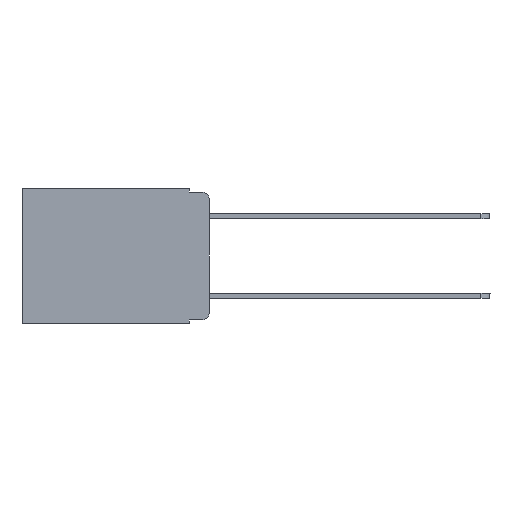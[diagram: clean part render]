
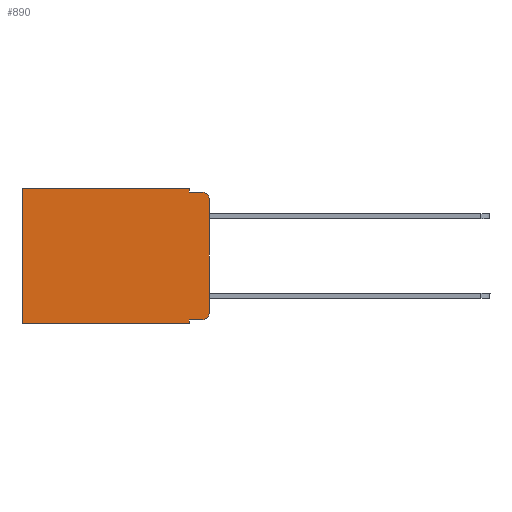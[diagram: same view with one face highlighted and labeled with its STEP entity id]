
A CAD part, left-side view. The second image highlights one B-rep face of the part: STEP entity #890.
In plain terms, the highlighted planar face has unit normal (-1, 0, 0).
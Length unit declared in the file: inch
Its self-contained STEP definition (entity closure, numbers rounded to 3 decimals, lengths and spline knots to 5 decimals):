
#130 = VERTEX_POINT ( 'NONE', #11338 ) ;
#194 = EDGE_CURVE ( 'NONE', #1970, #130, #1797, .T. ) ;
#262 = CARTESIAN_POINT ( 'NONE',  ( 0.298, 0.051, -0.01 ) ) ;
#366 = CARTESIAN_POINT ( 'NONE',  ( 0.298, 0.02, -0.333 ) ) ;
#757 = CARTESIAN_POINT ( 'NONE',  ( 0.298, 0.02, -0.03 ) ) ;
#767 = AXIS2_PLACEMENT_3D ( 'NONE', #757, #12430, #4545 ) ;
#769 = VERTEX_POINT ( 'NONE', #12163 ) ;
#771 = EDGE_CURVE ( 'NONE', #1970, #4406, #1932, .T. ) ;
#853 = CARTESIAN_POINT ( 'NONE',  ( 0.298, 0.051, -0.333 ) ) ;
#890 = ADVANCED_FACE ( 'NONE', ( #1318 ), #4174, .F. ) ;
#947 = ORIENTED_EDGE ( 'NONE', *, *, #4302, .F. ) ;
#1174 = VERTEX_POINT ( 'NONE', #366 ) ;
#1262 = EDGE_CURVE ( 'NONE', #769, #4809, #11128, .T. ) ;
#1296 = DIRECTION ( 'NONE',  ( 1., 0., 0. ) ) ;
#1318 = FACE_OUTER_BOUND ( 'NONE', #2190, .T. ) ;
#1337 = DIRECTION ( 'NONE',  ( 0., -1., 0. ) ) ;
#1653 = DIRECTION ( 'NONE',  ( 0., 0., -1. ) ) ;
#1671 = CARTESIAN_POINT ( 'NONE',  ( 0.298, 0.051, -0.333 ) ) ;
#1688 = CARTESIAN_POINT ( 'NONE',  ( 0.298, 0.051, 0. ) ) ;
#1797 = CIRCLE ( 'NONE', #767, 0.02 ) ;
#1932 = LINE ( 'NONE', #9241, #8735 ) ;
#1970 = VERTEX_POINT ( 'NONE', #4119 ) ;
#1990 = ORIENTED_EDGE ( 'NONE', *, *, #4877, .T. ) ;
#2064 = DIRECTION ( 'NONE',  ( 0., 0., -1. ) ) ;
#2074 = EDGE_CURVE ( 'NONE', #4519, #8644, #9302, .T. ) ;
#2190 = EDGE_LOOP ( 'NONE', ( #9070, #6346, #947, #5321, #1990, #2446, #9105, #8401, #3474, #5586 ) ) ;
#2446 = ORIENTED_EDGE ( 'NONE', *, *, #2074, .T. ) ;
#2481 = CARTESIAN_POINT ( 'NONE',  ( 0.298, 0.051, -0.01 ) ) ;
#2931 = CARTESIAN_POINT ( 'NONE',  ( 0.298, 0., 0. ) ) ;
#3101 = VECTOR ( 'NONE', #9969, 39.37008 ) ;
#3474 = ORIENTED_EDGE ( 'NONE', *, *, #5891, .T. ) ;
#4039 = DIRECTION ( 'NONE',  ( 0., 1., 0. ) ) ;
#4119 = CARTESIAN_POINT ( 'NONE',  ( 0.298, 0., -0.03 ) ) ;
#4174 = PLANE ( 'NONE',  #6075 ) ;
#4302 = EDGE_CURVE ( 'NONE', #4809, #130, #10733, .T. ) ;
#4406 = VERTEX_POINT ( 'NONE', #6830 ) ;
#4420 = DIRECTION ( 'NONE',  ( 0., 0., -1. ) ) ;
#4519 = VERTEX_POINT ( 'NONE', #7406 ) ;
#4545 = DIRECTION ( 'NONE',  ( 0., 0., -1. ) ) ;
#4728 = CARTESIAN_POINT ( 'NONE',  ( 0.298, 0.02, -0.313 ) ) ;
#4809 = VERTEX_POINT ( 'NONE', #262 ) ;
#4877 = EDGE_CURVE ( 'NONE', #769, #4519, #11783, .T. ) ;
#5139 = VERTEX_POINT ( 'NONE', #853 ) ;
#5321 = ORIENTED_EDGE ( 'NONE', *, *, #1262, .F. ) ;
#5505 = DIRECTION ( 'NONE',  ( 0., -1., 0. ) ) ;
#5561 = LINE ( 'NONE', #1688, #10544 ) ;
#5586 = ORIENTED_EDGE ( 'NONE', *, *, #9792, .T. ) ;
#5710 = CIRCLE ( 'NONE', #6623, 0.02 ) ;
#5865 = VECTOR ( 'NONE', #5505, 39.37008 ) ;
#5891 = EDGE_CURVE ( 'NONE', #5139, #1174, #10093, .T. ) ;
#5900 = CARTESIAN_POINT ( 'NONE',  ( 0.298, 0.051, 0. ) ) ;
#6075 = AXIS2_PLACEMENT_3D ( 'NONE', #2931, #1296, #2064 ) ;
#6346 = ORIENTED_EDGE ( 'NONE', *, *, #194, .T. ) ;
#6623 = AXIS2_PLACEMENT_3D ( 'NONE', #4728, #12495, #11435 ) ;
#6828 = VECTOR ( 'NONE', #1337, 39.37008 ) ;
#6830 = CARTESIAN_POINT ( 'NONE',  ( 0.298, 0., -0.313 ) ) ;
#7376 = VECTOR ( 'NONE', #8666, 39.37008 ) ;
#7406 = CARTESIAN_POINT ( 'NONE',  ( 0.298, 0.473, 0. ) ) ;
#8332 = DIRECTION ( 'NONE',  ( 0., 0., -1. ) ) ;
#8345 = CARTESIAN_POINT ( 'NONE',  ( 0.298, 0.051, -0.343 ) ) ;
#8401 = ORIENTED_EDGE ( 'NONE', *, *, #9256, .F. ) ;
#8502 = CARTESIAN_POINT ( 'NONE',  ( 0.298, 0.473, -0.343 ) ) ;
#8589 = VERTEX_POINT ( 'NONE', #8345 ) ;
#8644 = VERTEX_POINT ( 'NONE', #8502 ) ;
#8666 = DIRECTION ( 'NONE',  ( 0., 0., -1. ) ) ;
#8735 = VECTOR ( 'NONE', #1653, 39.37008 ) ;
#8901 = CARTESIAN_POINT ( 'NONE',  ( 0.298, 0., 0. ) ) ;
#9070 = ORIENTED_EDGE ( 'NONE', *, *, #771, .F. ) ;
#9105 = ORIENTED_EDGE ( 'NONE', *, *, #10756, .F. ) ;
#9241 = CARTESIAN_POINT ( 'NONE',  ( 0.298, 0., 0. ) ) ;
#9256 = EDGE_CURVE ( 'NONE', #5139, #8589, #5561, .T. ) ;
#9302 = LINE ( 'NONE', #9944, #11575 ) ;
#9450 = LINE ( 'NONE', #10900, #3101 ) ;
#9792 = EDGE_CURVE ( 'NONE', #1174, #4406, #5710, .T. ) ;
#9944 = CARTESIAN_POINT ( 'NONE',  ( 0.298, 0.473, 0. ) ) ;
#9969 = DIRECTION ( 'NONE',  ( 0., 1., 0. ) ) ;
#10093 = LINE ( 'NONE', #1671, #5865 ) ;
#10269 = VECTOR ( 'NONE', #4039, 39.37008 ) ;
#10544 = VECTOR ( 'NONE', #8332, 39.37008 ) ;
#10733 = LINE ( 'NONE', #2481, #6828 ) ;
#10756 = EDGE_CURVE ( 'NONE', #8589, #8644, #9450, .T. ) ;
#10900 = CARTESIAN_POINT ( 'NONE',  ( 0.298, 0., -0.343 ) ) ;
#11128 = LINE ( 'NONE', #5900, #7376 ) ;
#11338 = CARTESIAN_POINT ( 'NONE',  ( 0.298, 0.02, -0.01 ) ) ;
#11435 = DIRECTION ( 'NONE',  ( 0., 0., -1. ) ) ;
#11575 = VECTOR ( 'NONE', #4420, 39.37008 ) ;
#11783 = LINE ( 'NONE', #8901, #10269 ) ;
#12163 = CARTESIAN_POINT ( 'NONE',  ( 0.298, 0.051, 0. ) ) ;
#12430 = DIRECTION ( 'NONE',  ( -1., 0., 0. ) ) ;
#12495 = DIRECTION ( 'NONE',  ( -1., 0., 0. ) ) ;
